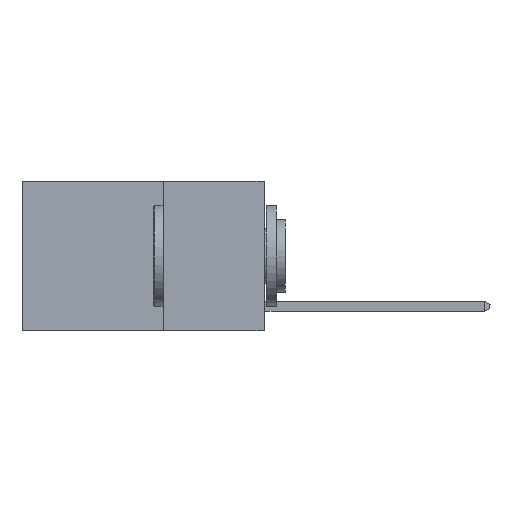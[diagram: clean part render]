
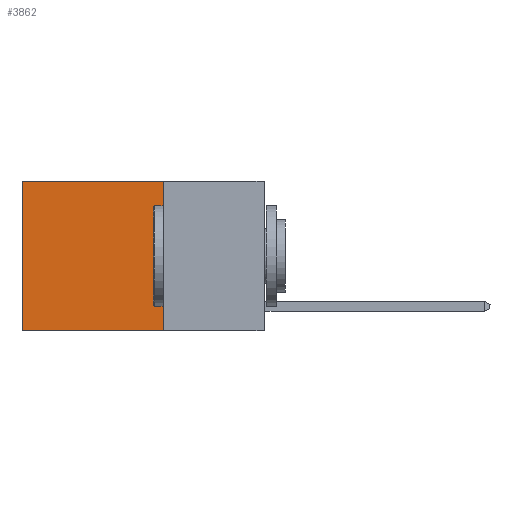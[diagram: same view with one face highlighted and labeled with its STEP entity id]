
A CAD part, left-side view. The second image highlights one B-rep face of the part: STEP entity #3862.
In plain terms, the highlighted planar face has unit normal (-1, 0, 0).
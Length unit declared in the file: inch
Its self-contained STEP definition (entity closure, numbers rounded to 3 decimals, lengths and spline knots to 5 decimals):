
#968 = VERTEX_POINT ( 'NONE', #23981 ) ;
#1635 = LINE ( 'NONE', #15500, #10351 ) ;
#1775 = CARTESIAN_POINT ( 'NONE',  ( 0.2625, 0.25, 0. ) ) ;
#2290 = ORIENTED_EDGE ( 'NONE', *, *, #21380, .T. ) ;
#3080 = LINE ( 'NONE', #1775, #8404 ) ;
#3141 = CARTESIAN_POINT ( 'NONE',  ( 0.2625, 0.25, -0.37 ) ) ;
#3862 = ADVANCED_FACE ( 'NONE', ( #6102 ), #5190, .F. ) ;
#5190 = PLANE ( 'NONE',  #25016 ) ;
#5598 = DIRECTION ( 'NONE',  ( 0., 0., -1. ) ) ;
#6100 = CARTESIAN_POINT ( 'NONE',  ( 0.2625, 0.25, 0. ) ) ;
#6102 = FACE_OUTER_BOUND ( 'NONE', #14896, .T. ) ;
#6578 = CARTESIAN_POINT ( 'NONE',  ( 0.2625, 0.25, 0. ) ) ;
#7199 = DIRECTION ( 'NONE',  ( 0., 0., -1. ) ) ;
#8404 = VECTOR ( 'NONE', #15687, 39.37008 ) ;
#9075 = DIRECTION ( 'NONE',  ( 0., 1., 0. ) ) ;
#10351 = VECTOR ( 'NONE', #5598, 39.37008 ) ;
#10928 = CARTESIAN_POINT ( 'NONE',  ( 0.2625, 0.6, -0.37 ) ) ;
#11267 = CARTESIAN_POINT ( 'NONE',  ( 0.2625, 0.25, -0.37 ) ) ;
#11711 = LINE ( 'NONE', #3141, #16374 ) ;
#12534 = ORIENTED_EDGE ( 'NONE', *, *, #13889, .F. ) ;
#13117 = VERTEX_POINT ( 'NONE', #6578 ) ;
#13889 = EDGE_CURVE ( 'NONE', #13117, #19922, #3080, .T. ) ;
#14199 = VECTOR ( 'NONE', #19969, 39.37008 ) ;
#14896 = EDGE_LOOP ( 'NONE', ( #23287, #24191, #12534, #2290 ) ) ;
#15500 = CARTESIAN_POINT ( 'NONE',  ( 0.2625, 0.6, 0. ) ) ;
#15687 = DIRECTION ( 'NONE',  ( 0., 0., -1. ) ) ;
#16374 = VECTOR ( 'NONE', #9075, 39.37008 ) ;
#17983 = EDGE_CURVE ( 'NONE', #968, #18990, #1635, .T. ) ;
#18990 = VERTEX_POINT ( 'NONE', #10928 ) ;
#19069 = DIRECTION ( 'NONE',  ( 1., 0., 0. ) ) ;
#19922 = VERTEX_POINT ( 'NONE', #11267 ) ;
#19969 = DIRECTION ( 'NONE',  ( 0., 1., 0. ) ) ;
#21078 = EDGE_CURVE ( 'NONE', #19922, #18990, #11711, .T. ) ;
#21380 = EDGE_CURVE ( 'NONE', #13117, #968, #24711, .T. ) ;
#23287 = ORIENTED_EDGE ( 'NONE', *, *, #17983, .T. ) ;
#23981 = CARTESIAN_POINT ( 'NONE',  ( 0.2625, 0.6, 0. ) ) ;
#24191 = ORIENTED_EDGE ( 'NONE', *, *, #21078, .F. ) ;
#24711 = LINE ( 'NONE', #6100, #14199 ) ;
#24950 = CARTESIAN_POINT ( 'NONE',  ( 0.2625, 0.25, 0. ) ) ;
#25016 = AXIS2_PLACEMENT_3D ( 'NONE', #24950, #19069, #7199 ) ;
